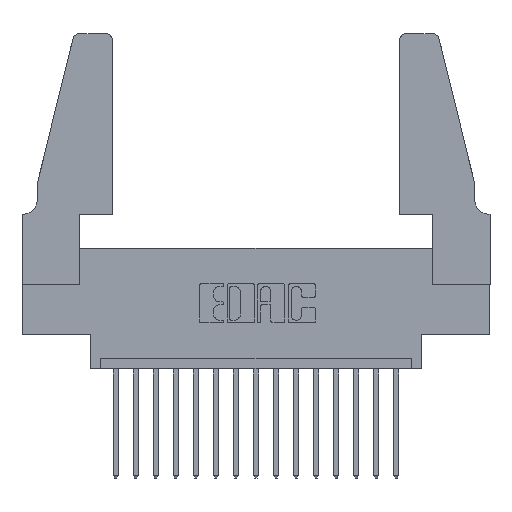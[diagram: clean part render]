
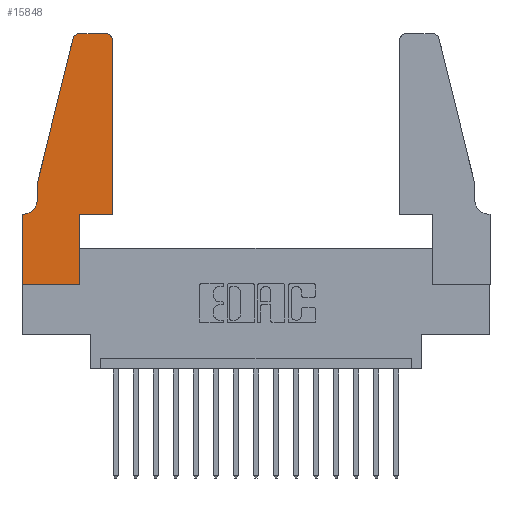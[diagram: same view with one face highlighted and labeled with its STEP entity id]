
A CAD part, top view. The second image highlights one B-rep face of the part: STEP entity #15848.
In plain terms, the highlighted planar face has unit normal (0, 0, 1).
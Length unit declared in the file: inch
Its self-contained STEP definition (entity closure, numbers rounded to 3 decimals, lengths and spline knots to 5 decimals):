
#63 = CARTESIAN_POINT ( 'NONE',  ( 0.4505, 0.35, 0.37 ) ) ;
#74 = ORIENTED_EDGE ( 'NONE', *, *, #6744, .T. ) ;
#87 = VERTEX_POINT ( 'NONE', #946 ) ;
#155 = AXIS2_PLACEMENT_3D ( 'NONE', #9466, #12193, #10913 ) ;
#344 = FACE_OUTER_BOUND ( 'NONE', #13367, .T. ) ;
#497 = CIRCLE ( 'NONE', #2870, 0.03 ) ;
#946 = CARTESIAN_POINT ( 'NONE',  ( 0., 0.35, 0.37 ) ) ;
#1096 = VERTEX_POINT ( 'NONE', #8572 ) ;
#1270 = DIRECTION ( 'NONE',  ( 0., 0., 1. ) ) ;
#1323 = CARTESIAN_POINT ( 'NONE',  ( 0.0755, 0.5, 0.37 ) ) ;
#1438 = DIRECTION ( 'NONE',  ( -0.239, -0.971, 0. ) ) ;
#1750 = VERTEX_POINT ( 'NONE', #5321 ) ;
#1867 = CARTESIAN_POINT ( 'NONE',  ( 0.0755, 0.42, 0.37 ) ) ;
#1914 = VERTEX_POINT ( 'NONE', #10478 ) ;
#2021 = VECTOR ( 'NONE', #3985, 39.37008 ) ;
#2185 = EDGE_CURVE ( 'NONE', #3550, #12025, #16450, .T. ) ;
#2431 = LINE ( 'NONE', #63, #2021 ) ;
#2870 = AXIS2_PLACEMENT_3D ( 'NONE', #17197, #1270, #11966 ) ;
#3148 = VERTEX_POINT ( 'NONE', #12786 ) ;
#3449 = LINE ( 'NONE', #1323, #12019 ) ;
#3550 = VERTEX_POINT ( 'NONE', #1867 ) ;
#3754 = DIRECTION ( 'NONE',  ( 0., 0., 1. ) ) ;
#3783 = VERTEX_POINT ( 'NONE', #14739 ) ;
#3807 = PLANE ( 'NONE',  #10718 ) ;
#3985 = DIRECTION ( 'NONE',  ( 1., 0., 0. ) ) ;
#4278 = CARTESIAN_POINT ( 'NONE',  ( 0.0055, 0.35, 0.37 ) ) ;
#4771 = EDGE_CURVE ( 'NONE', #1914, #14887, #2431, .T. ) ;
#4793 = CIRCLE ( 'NONE', #155, 0.03 ) ;
#4854 = ORIENTED_EDGE ( 'NONE', *, *, #14421, .T. ) ;
#4954 = ORIENTED_EDGE ( 'NONE', *, *, #13740, .T. ) ;
#5289 = DIRECTION ( 'NONE',  ( -1., 0., 0. ) ) ;
#5321 = CARTESIAN_POINT ( 'NONE',  ( 0., 0., 0.37 ) ) ;
#5507 = CARTESIAN_POINT ( 'NONE',  ( 0.4505, 1.22, 0.37 ) ) ;
#5614 = CARTESIAN_POINT ( 'NONE',  ( 0.0755, 0.5, 0.37 ) ) ;
#5693 = DIRECTION ( 'NONE',  ( -1., 0., 0. ) ) ;
#5837 = LINE ( 'NONE', #12474, #6879 ) ;
#5849 = ORIENTED_EDGE ( 'NONE', *, *, #2185, .T. ) ;
#5928 = EDGE_CURVE ( 'NONE', #1750, #3148, #9093, .T. ) ;
#6744 = EDGE_CURVE ( 'NONE', #87, #1750, #7172, .T. ) ;
#6796 = AXIS2_PLACEMENT_3D ( 'NONE', #14893, #16267, #5693 ) ;
#6879 = VECTOR ( 'NONE', #12415, 39.37008 ) ;
#7172 = LINE ( 'NONE', #15882, #17137 ) ;
#7247 = ORIENTED_EDGE ( 'NONE', *, *, #17035, .T. ) ;
#7514 = VECTOR ( 'NONE', #10997, 39.37008 ) ;
#7926 = DIRECTION ( 'NONE',  ( 0., -1., 0. ) ) ;
#8247 = VERTEX_POINT ( 'NONE', #15916 ) ;
#8572 = CARTESIAN_POINT ( 'NONE',  ( 0.4205, 1.25, 0.37 ) ) ;
#9093 = LINE ( 'NONE', #12805, #11601 ) ;
#9466 = CARTESIAN_POINT ( 'NONE',  ( 0.284, 1.22, 0.37 ) ) ;
#9625 = LINE ( 'NONE', #10197, #13988 ) ;
#9852 = ORIENTED_EDGE ( 'NONE', *, *, #17118, .T. ) ;
#9881 = CARTESIAN_POINT ( 'NONE',  ( 0.0755, 0.35, 0.37 ) ) ;
#10026 = DIRECTION ( 'NONE',  ( -1., 0., 0. ) ) ;
#10197 = CARTESIAN_POINT ( 'NONE',  ( 0.2605, 1.25, 0.37 ) ) ;
#10478 = CARTESIAN_POINT ( 'NONE',  ( 0.2865, 0.35, 0.37 ) ) ;
#10680 = VERTEX_POINT ( 'NONE', #5507 ) ;
#10718 = AXIS2_PLACEMENT_3D ( 'NONE', #11780, #3754, #13090 ) ;
#10874 = CARTESIAN_POINT ( 'NONE',  ( 0.4505, 0.35, 0.37 ) ) ;
#10913 = DIRECTION ( 'NONE',  ( 1., 0., 0. ) ) ;
#10997 = DIRECTION ( 'NONE',  ( 0., 1., 0. ) ) ;
#11357 = EDGE_CURVE ( 'NONE', #1096, #8247, #9625, .T. ) ;
#11562 = ORIENTED_EDGE ( 'NONE', *, *, #11357, .T. ) ;
#11601 = VECTOR ( 'NONE', #14122, 39.37008 ) ;
#11780 = CARTESIAN_POINT ( 'NONE',  ( 0., 0.35, 0.37 ) ) ;
#11805 = EDGE_CURVE ( 'NONE', #3148, #1914, #5837, .T. ) ;
#11966 = DIRECTION ( 'NONE',  ( 1., 0., 0. ) ) ;
#12019 = VECTOR ( 'NONE', #1438, 39.37008 ) ;
#12025 = VERTEX_POINT ( 'NONE', #4278 ) ;
#12193 = DIRECTION ( 'NONE',  ( 0., 0., 1. ) ) ;
#12415 = DIRECTION ( 'NONE',  ( 0., 1., 0. ) ) ;
#12474 = CARTESIAN_POINT ( 'NONE',  ( 0.2865, 0.35, 0.37 ) ) ;
#12786 = CARTESIAN_POINT ( 'NONE',  ( 0.2865, 0., 0.37 ) ) ;
#12805 = CARTESIAN_POINT ( 'NONE',  ( 0., 0., 0.37 ) ) ;
#12815 = ORIENTED_EDGE ( 'NONE', *, *, #11805, .T. ) ;
#13090 = DIRECTION ( 'NONE',  ( 1., 0., 0. ) ) ;
#13158 = VERTEX_POINT ( 'NONE', #5614 ) ;
#13254 = CARTESIAN_POINT ( 'NONE',  ( 0.0755, 0.5, 0.37 ) ) ;
#13367 = EDGE_LOOP ( 'NONE', ( #11562, #4954, #9852, #4854, #5849, #16434, #74, #16588, #12815, #16935, #15067, #7247 ) ) ;
#13740 = EDGE_CURVE ( 'NONE', #8247, #3783, #4793, .T. ) ;
#13955 = LINE ( 'NONE', #9881, #14354 ) ;
#13988 = VECTOR ( 'NONE', #10026, 39.37008 ) ;
#14122 = DIRECTION ( 'NONE',  ( 1., 0., 0. ) ) ;
#14354 = VECTOR ( 'NONE', #5289, 39.37008 ) ;
#14371 = LINE ( 'NONE', #10874, #7514 ) ;
#14421 = EDGE_CURVE ( 'NONE', #13158, #3550, #16842, .T. ) ;
#14654 = EDGE_CURVE ( 'NONE', #14887, #10680, #14371, .T. ) ;
#14739 = CARTESIAN_POINT ( 'NONE',  ( 0.25487, 1.22718, 0.37 ) ) ;
#14887 = VERTEX_POINT ( 'NONE', #16571 ) ;
#14893 = CARTESIAN_POINT ( 'NONE',  ( 0.0055, 0.42, 0.37 ) ) ;
#15067 = ORIENTED_EDGE ( 'NONE', *, *, #14654, .T. ) ;
#15292 = EDGE_CURVE ( 'NONE', #12025, #87, #13955, .T. ) ;
#15848 = ADVANCED_FACE ( 'NONE', ( #344 ), #3807, .T. ) ;
#15882 = CARTESIAN_POINT ( 'NONE',  ( 0., 0., 0.37 ) ) ;
#15916 = CARTESIAN_POINT ( 'NONE',  ( 0.284, 1.25, 0.37 ) ) ;
#16023 = VECTOR ( 'NONE', #16346, 39.37008 ) ;
#16267 = DIRECTION ( 'NONE',  ( 0., 0., -1. ) ) ;
#16346 = DIRECTION ( 'NONE',  ( 0., -1., 0. ) ) ;
#16434 = ORIENTED_EDGE ( 'NONE', *, *, #15292, .T. ) ;
#16450 = CIRCLE ( 'NONE', #6796, 0.07 ) ;
#16571 = CARTESIAN_POINT ( 'NONE',  ( 0.4505, 0.35, 0.37 ) ) ;
#16588 = ORIENTED_EDGE ( 'NONE', *, *, #5928, .T. ) ;
#16842 = LINE ( 'NONE', #13254, #16023 ) ;
#16935 = ORIENTED_EDGE ( 'NONE', *, *, #4771, .T. ) ;
#17035 = EDGE_CURVE ( 'NONE', #10680, #1096, #497, .T. ) ;
#17118 = EDGE_CURVE ( 'NONE', #3783, #13158, #3449, .T. ) ;
#17137 = VECTOR ( 'NONE', #7926, 39.37008 ) ;
#17197 = CARTESIAN_POINT ( 'NONE',  ( 0.4205, 1.22, 0.37 ) ) ;
